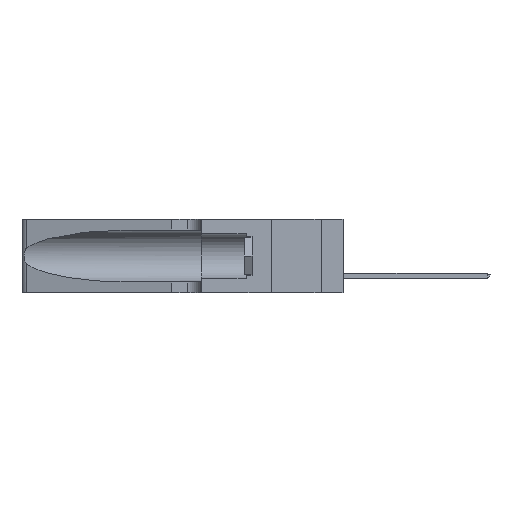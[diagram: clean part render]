
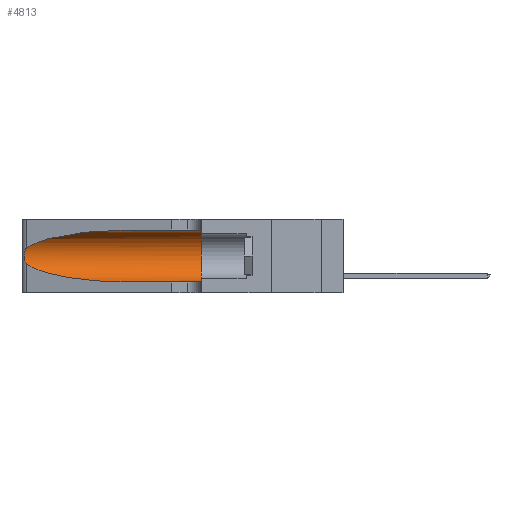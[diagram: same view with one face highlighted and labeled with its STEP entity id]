
A CAD part, left-side view. The second image highlights one B-rep face of the part: STEP entity #4813.
In plain terms, the highlighted cylindrical face has radius 3.308 mm (diameter 6.617 mm), a partial arc.
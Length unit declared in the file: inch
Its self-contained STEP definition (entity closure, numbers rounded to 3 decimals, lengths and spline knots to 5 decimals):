
#15 = EDGE_CURVE ( 'NONE', #26145, #7693, #6512, .T. ) ;
#145 = CARTESIAN_POINT ( 'NONE',  ( 0.25555, 1.22994, 0.2215 ) ) ;
#283 =( BOUNDED_CURVE ( )  B_SPLINE_CURVE ( 3, ( #6573, #9126, #30167, #17084 ),
 .UNSPECIFIED., .F., .T. ) 
 B_SPLINE_CURVE_WITH_KNOTS ( ( 4, 4 ),
 ( 1.5708, 2.84003 ),
 .UNSPECIFIED. ) 
 CURVE ( )  GEOMETRIC_REPRESENTATION_ITEM ( )  RATIONAL_B_SPLINE_CURVE ( ( 1., 0.87, 0.87, 1. ) ) 
 REPRESENTATION_ITEM ( '' )  );
#1968 = EDGE_CURVE ( 'NONE', #19744, #23630, #31668, .T. ) ;
#2528 = DIRECTION ( 'NONE',  ( 0., -1., 0. ) ) ;
#3315 = CARTESIAN_POINT ( 'NONE',  ( 0.25856, 1.23593, 0.16098 ) ) ;
#3536 = CARTESIAN_POINT ( 'NONE',  ( 0.18966, 0.96281, 0.05475 ) ) ;
#3577 = CARTESIAN_POINT ( 'NONE',  ( 0.1305, 0.72297, 0.05475 ) ) ;
#3854 = DIRECTION ( 'NONE',  ( 0., -1., 0. ) ) ;
#4055 = VERTEX_POINT ( 'NONE', #25932 ) ;
#4813 = ADVANCED_FACE ( 'NONE', ( #19055 ), #12074, .F. ) ;
#5719 = CARTESIAN_POINT ( 'NONE',  ( 0.25639, 1.23184, 0.21858 ) ) ;
#5804 = EDGE_CURVE ( 'NONE', #4055, #26145, #283, .T. ) ;
#6288 = CARTESIAN_POINT ( 'NONE',  ( 0.1305, 0.35, 0.185 ) ) ;
#6512 = B_SPLINE_CURVE_WITH_KNOTS ( 'NONE', 3,
 ( #21539, #145, #5719, #8373, #18631, #26617, #26824, #15770, #34351, #3315, #18722, #21399, #11361, #13984 ),
 .UNSPECIFIED., .F., .F.,
 ( 4, 2, 2, 2, 2, 2, 4 ),
 ( 0., 0.00027, 0.00053, 0.00107, 0.0016, 0.00187, 0.00214 ),
 .UNSPECIFIED. ) ;
#6573 = CARTESIAN_POINT ( 'NONE',  ( 0.1305, 0.72297, 0.31525 ) ) ;
#6679 = EDGE_CURVE ( 'NONE', #33263, #23630, #32743, .T. ) ;
#7693 = VERTEX_POINT ( 'NONE', #11080 ) ;
#7881 = EDGE_CURVE ( 'NONE', #4055, #19744, #9871, .T. ) ;
#8373 = CARTESIAN_POINT ( 'NONE',  ( 0.25787, 1.23484, 0.2124 ) ) ;
#8936 = CARTESIAN_POINT ( 'NONE',  ( 0.2373, 1.15595, 0.08982 ) ) ;
#9126 = CARTESIAN_POINT ( 'NONE',  ( 0.18966, 0.96281, 0.31525 ) ) ;
#9871 = LINE ( 'NONE', #20172, #16033 ) ;
#11080 = CARTESIAN_POINT ( 'NONE',  ( 0.25487, 1.22718, 0.14631 ) ) ;
#11357 = CARTESIAN_POINT ( 'NONE',  ( 0.1305, 0.72297, 0.05475 ) ) ;
#11361 = CARTESIAN_POINT ( 'NONE',  ( 0.25555, 1.22993, 0.14849 ) ) ;
#11698 = CARTESIAN_POINT ( 'NONE',  ( 0.25487, 1.22718, 0.14631 ) ) ;
#12074 = CYLINDRICAL_SURFACE ( 'NONE', #33193, 0.13025 ) ;
#13203 = CARTESIAN_POINT ( 'NONE',  ( 0.1305, 1.61858, 0.185 ) ) ;
#13822 = CARTESIAN_POINT ( 'NONE',  ( 0.25487, 1.22718, 0.22369 ) ) ;
#13947 = ORIENTED_EDGE ( 'NONE', *, *, #29988, .T. ) ;
#13984 = CARTESIAN_POINT ( 'NONE',  ( 0.25487, 1.22718, 0.14631 ) ) ;
#15770 = CARTESIAN_POINT ( 'NONE',  ( 0.26075, 1.23896, 0.178 ) ) ;
#16033 = VECTOR ( 'NONE', #25373, 39.37008 ) ;
#17084 = CARTESIAN_POINT ( 'NONE',  ( 0.25487, 1.22718, 0.22369 ) ) ;
#18631 = CARTESIAN_POINT ( 'NONE',  ( 0.25854, 1.2359, 0.20912 ) ) ;
#18722 = CARTESIAN_POINT ( 'NONE',  ( 0.25789, 1.23486, 0.15765 ) ) ;
#19055 = FACE_OUTER_BOUND ( 'NONE', #25409, .T. ) ;
#19395 = CARTESIAN_POINT ( 'NONE',  ( 0.1305, 0.35, 0.31525 ) ) ;
#19436 = VECTOR ( 'NONE', #2528, 39.37008 ) ;
#19744 = VERTEX_POINT ( 'NONE', #19395 ) ;
#19771 = DIRECTION ( 'NONE',  ( 0., 0., 1. ) ) ;
#20081 = DIRECTION ( 'NONE',  ( 0., 0., -1. ) ) ;
#20172 = CARTESIAN_POINT ( 'NONE',  ( 0.1305, 1.61858, 0.31525 ) ) ;
#20758 = ORIENTED_EDGE ( 'NONE', *, *, #1968, .F. ) ;
#21399 = CARTESIAN_POINT ( 'NONE',  ( 0.25639, 1.23186, 0.15144 ) ) ;
#21539 = CARTESIAN_POINT ( 'NONE',  ( 0.25487, 1.22718, 0.22369 ) ) ;
#21692 = ORIENTED_EDGE ( 'NONE', *, *, #7881, .F. ) ;
#22487 = AXIS2_PLACEMENT_3D ( 'NONE', #6288, #24740, #19771 ) ;
#23041 = ORIENTED_EDGE ( 'NONE', *, *, #15, .T. ) ;
#23630 = VERTEX_POINT ( 'NONE', #32137 ) ;
#23901 = ORIENTED_EDGE ( 'NONE', *, *, #5804, .T. ) ;
#24740 = DIRECTION ( 'NONE',  ( 0., 1., 0. ) ) ;
#25373 = DIRECTION ( 'NONE',  ( 0., -1., 0. ) ) ;
#25409 = EDGE_LOOP ( 'NONE', ( #23901, #23041, #13947, #26542, #20758, #21692 ) ) ;
#25932 = CARTESIAN_POINT ( 'NONE',  ( 0.1305, 0.72297, 0.31525 ) ) ;
#26145 = VERTEX_POINT ( 'NONE', #13822 ) ;
#26387 = CARTESIAN_POINT ( 'NONE',  ( 0.1305, 1.61858, 0.05475 ) ) ;
#26542 = ORIENTED_EDGE ( 'NONE', *, *, #6679, .T. ) ;
#26617 = CARTESIAN_POINT ( 'NONE',  ( 0.26018, 1.23835, 0.19895 ) ) ;
#26824 = CARTESIAN_POINT ( 'NONE',  ( 0.26075, 1.23896, 0.19203 ) ) ;
#28091 =( BOUNDED_CURVE ( )  B_SPLINE_CURVE ( 3, ( #11698, #8936, #3536, #11357 ),
 .UNSPECIFIED., .F., .F. ) 
 B_SPLINE_CURVE_WITH_KNOTS ( ( 4, 4 ),
 ( 3.44316, 4.71239 ),
 .UNSPECIFIED. ) 
 CURVE ( )  GEOMETRIC_REPRESENTATION_ITEM ( )  RATIONAL_B_SPLINE_CURVE ( ( 1., 0.87, 0.87, 1. ) ) 
 REPRESENTATION_ITEM ( '' )  );
#29988 = EDGE_CURVE ( 'NONE', #7693, #33263, #28091, .T. ) ;
#30167 = CARTESIAN_POINT ( 'NONE',  ( 0.2373, 1.15595, 0.28018 ) ) ;
#31668 = CIRCLE ( 'NONE', #22487, 0.13025 ) ;
#32137 = CARTESIAN_POINT ( 'NONE',  ( 0.1305, 0.35, 0.05475 ) ) ;
#32743 = LINE ( 'NONE', #26387, #19436 ) ;
#33193 = AXIS2_PLACEMENT_3D ( 'NONE', #13203, #3854, #20081 ) ;
#33263 = VERTEX_POINT ( 'NONE', #3577 ) ;
#34351 = CARTESIAN_POINT ( 'NONE',  ( 0.26017, 1.23833, 0.17102 ) ) ;
